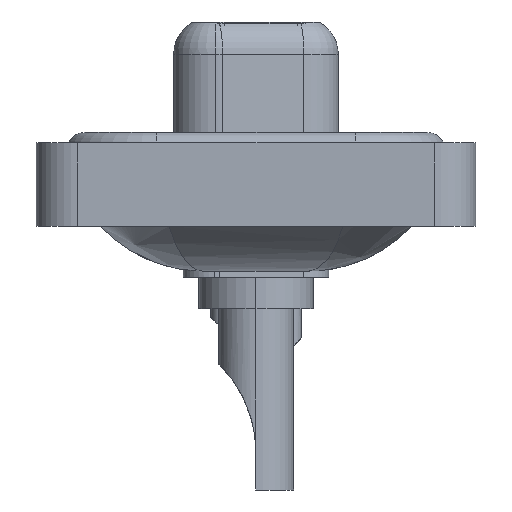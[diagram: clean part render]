
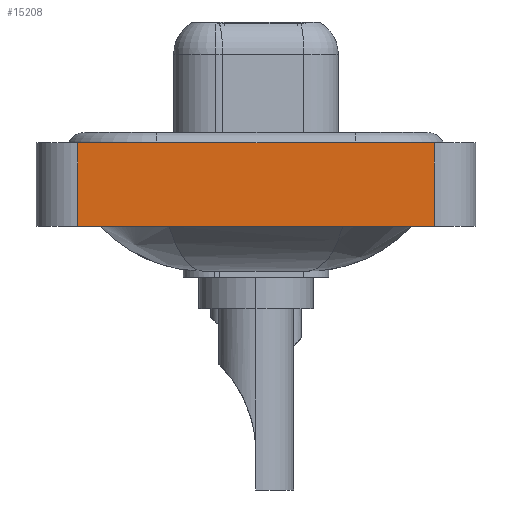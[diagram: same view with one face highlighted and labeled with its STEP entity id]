
A CAD part, left-side view. The second image highlights one B-rep face of the part: STEP entity #15208.
In plain terms, the highlighted planar face has unit normal (-1, 0, 0).
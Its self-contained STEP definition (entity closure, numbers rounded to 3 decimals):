
#655 = VECTOR ( 'NONE', #14181, 1000. ) ;
#825 = LINE ( 'NONE', #1052, #12109 ) ;
#947 = LINE ( 'NONE', #9186, #655 ) ;
#1052 = CARTESIAN_POINT ( 'NONE',  ( -7.3, -8.55, -3.6 ) ) ;
#1415 = DIRECTION ( 'NONE',  ( 0., 0., 1. ) ) ;
#1723 = DIRECTION ( 'NONE',  ( 0., 0., 1. ) ) ;
#2536 = DIRECTION ( 'NONE',  ( 0., -1., 0. ) ) ;
#6469 = CARTESIAN_POINT ( 'NONE',  ( -7.3, -8.55, -3.6 ) ) ;
#6566 = PLANE ( 'NONE',  #18068 ) ;
#6737 = CARTESIAN_POINT ( 'NONE',  ( -7.3, -8.55, -3.6 ) ) ;
#6897 = ORIENTED_EDGE ( 'NONE', *, *, #8844, .F. ) ;
#7746 = EDGE_LOOP ( 'NONE', ( #12839, #6897, #17668, #13035 ) ) ;
#8844 = EDGE_CURVE ( 'NONE', #19951, #14291, #15597, .T. ) ;
#9186 = CARTESIAN_POINT ( 'NONE',  ( -7.3, 8.55, -3.6 ) ) ;
#9215 = CARTESIAN_POINT ( 'NONE',  ( -7.3, -8.55, 0.4 ) ) ;
#9789 = EDGE_CURVE ( 'NONE', #17685, #14291, #18480, .T. ) ;
#10862 = CARTESIAN_POINT ( 'NONE',  ( -7.3, -8.55, 0.4 ) ) ;
#11464 = DIRECTION ( 'NONE',  ( -1., 0., 0. ) ) ;
#12032 = CARTESIAN_POINT ( 'NONE',  ( -7.3, 8.55, -3.6 ) ) ;
#12109 = VECTOR ( 'NONE', #2536, 1000. ) ;
#12839 = ORIENTED_EDGE ( 'NONE', *, *, #9789, .T. ) ;
#13035 = ORIENTED_EDGE ( 'NONE', *, *, #18660, .T. ) ;
#14181 = DIRECTION ( 'NONE',  ( 0., 0., 1. ) ) ;
#14291 = VERTEX_POINT ( 'NONE', #10862 ) ;
#14488 = VECTOR ( 'NONE', #1415, 1000. ) ;
#14787 = VECTOR ( 'NONE', #18732, 1000. ) ;
#15208 = ADVANCED_FACE ( 'NONE', ( #20747 ), #6566, .T. ) ;
#15597 = LINE ( 'NONE', #9215, #14787 ) ;
#16487 = CARTESIAN_POINT ( 'NONE',  ( -7.3, 8.55, 0.4 ) ) ;
#17668 = ORIENTED_EDGE ( 'NONE', *, *, #18643, .F. ) ;
#17685 = VERTEX_POINT ( 'NONE', #6737 ) ;
#18068 = AXIS2_PLACEMENT_3D ( 'NONE', #6469, #11464, #1723 ) ;
#18480 = LINE ( 'NONE', #18684, #14488 ) ;
#18643 = EDGE_CURVE ( 'NONE', #20223, #19951, #947, .T. ) ;
#18660 = EDGE_CURVE ( 'NONE', #20223, #17685, #825, .T. ) ;
#18684 = CARTESIAN_POINT ( 'NONE',  ( -7.3, -8.55, -3.6 ) ) ;
#18732 = DIRECTION ( 'NONE',  ( 0., -1., 0. ) ) ;
#19951 = VERTEX_POINT ( 'NONE', #16487 ) ;
#20223 = VERTEX_POINT ( 'NONE', #12032 ) ;
#20747 = FACE_OUTER_BOUND ( 'NONE', #7746, .T. ) ;
